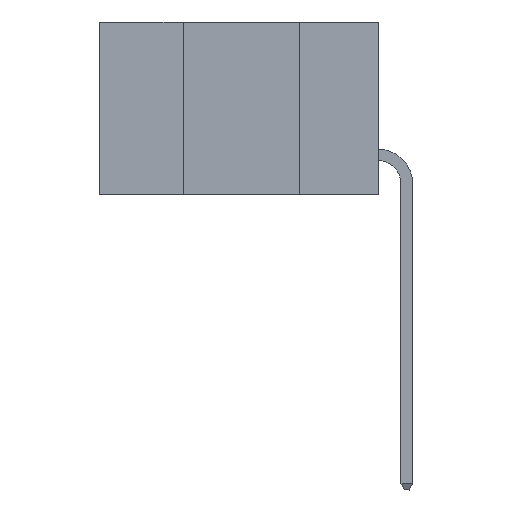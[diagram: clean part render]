
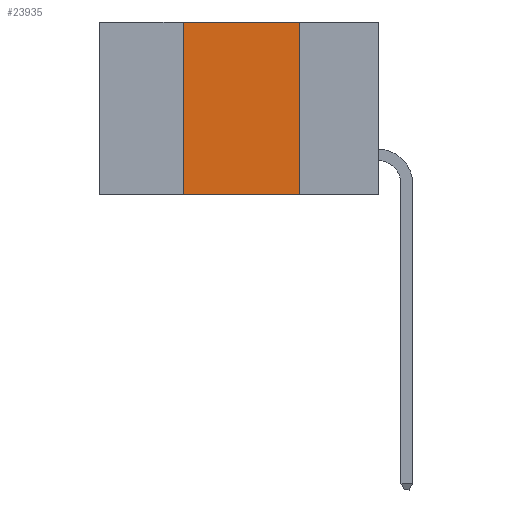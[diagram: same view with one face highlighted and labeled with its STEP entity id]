
A CAD part, left-side view. The second image highlights one B-rep face of the part: STEP entity #23935.
In plain terms, the highlighted planar face has unit normal (-1, 0, 0).
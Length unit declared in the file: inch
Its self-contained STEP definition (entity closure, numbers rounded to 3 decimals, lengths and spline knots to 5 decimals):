
#408 = VERTEX_POINT ( 'NONE', #23796 ) ;
#1701 = CARTESIAN_POINT ( 'NONE',  ( 0., 0.42, -0.37 ) ) ;
#1916 = VERTEX_POINT ( 'NONE', #14318 ) ;
#1969 = AXIS2_PLACEMENT_3D ( 'NONE', #18630, #5250, #20539 ) ;
#2277 = DIRECTION ( 'NONE',  ( 0., -1., 0. ) ) ;
#2718 = LINE ( 'NONE', #6116, #24613 ) ;
#3310 = FACE_OUTER_BOUND ( 'NONE', #15038, .T. ) ;
#3961 = LINE ( 'NONE', #11793, #15931 ) ;
#5250 = DIRECTION ( 'NONE',  ( 1., 0., 0. ) ) ;
#6116 = CARTESIAN_POINT ( 'NONE',  ( 0., 0.42, -0.37 ) ) ;
#6428 = ORIENTED_EDGE ( 'NONE', *, *, #16447, .F. ) ;
#9143 = ORIENTED_EDGE ( 'NONE', *, *, #13729, .T. ) ;
#9375 = CARTESIAN_POINT ( 'NONE',  ( 0., 0.17, -0.37 ) ) ;
#10096 = CARTESIAN_POINT ( 'NONE',  ( 0., 0.6, -0.37 ) ) ;
#11793 = CARTESIAN_POINT ( 'NONE',  ( 0., 0.6, 0. ) ) ;
#13729 = EDGE_CURVE ( 'NONE', #18048, #15493, #18085, .T. ) ;
#13950 = DIRECTION ( 'NONE',  ( 0., 0., 1. ) ) ;
#14318 = CARTESIAN_POINT ( 'NONE',  ( 0., 0.17, 0. ) ) ;
#14504 = EDGE_CURVE ( 'NONE', #1916, #15493, #19154, .T. ) ;
#15038 = EDGE_LOOP ( 'NONE', ( #15668, #23911, #6428, #9143 ) ) ;
#15493 = VERTEX_POINT ( 'NONE', #21963 ) ;
#15668 = ORIENTED_EDGE ( 'NONE', *, *, #14504, .F. ) ;
#15931 = VECTOR ( 'NONE', #2277, 39.37008 ) ;
#16447 = EDGE_CURVE ( 'NONE', #18048, #408, #2718, .T. ) ;
#17575 = VECTOR ( 'NONE', #22991, 39.37008 ) ;
#18048 = VERTEX_POINT ( 'NONE', #1701 ) ;
#18085 = LINE ( 'NONE', #10096, #21217 ) ;
#18630 = CARTESIAN_POINT ( 'NONE',  ( 0., 0.6, 0. ) ) ;
#19154 = LINE ( 'NONE', #9375, #17575 ) ;
#19620 = DIRECTION ( 'NONE',  ( 0., -1., 0. ) ) ;
#20539 = DIRECTION ( 'NONE',  ( 0., 0., -1. ) ) ;
#20778 = PLANE ( 'NONE',  #1969 ) ;
#21217 = VECTOR ( 'NONE', #19620, 39.37008 ) ;
#21806 = EDGE_CURVE ( 'NONE', #408, #1916, #3961, .T. ) ;
#21963 = CARTESIAN_POINT ( 'NONE',  ( 0., 0.17, -0.37 ) ) ;
#22991 = DIRECTION ( 'NONE',  ( 0., 0., -1. ) ) ;
#23796 = CARTESIAN_POINT ( 'NONE',  ( 0., 0.42, 0. ) ) ;
#23911 = ORIENTED_EDGE ( 'NONE', *, *, #21806, .F. ) ;
#23935 = ADVANCED_FACE ( 'NONE', ( #3310 ), #20778, .F. ) ;
#24613 = VECTOR ( 'NONE', #13950, 39.37008 ) ;
